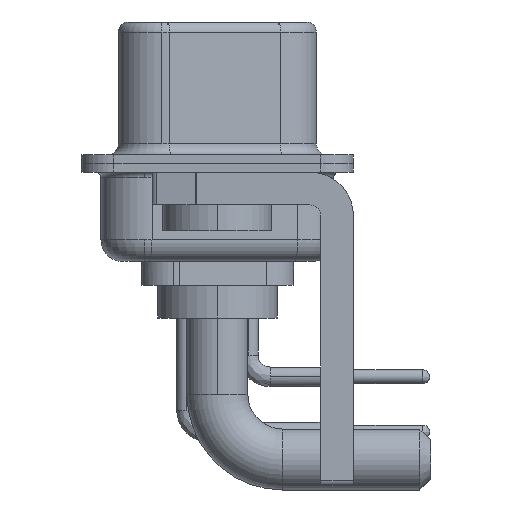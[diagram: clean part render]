
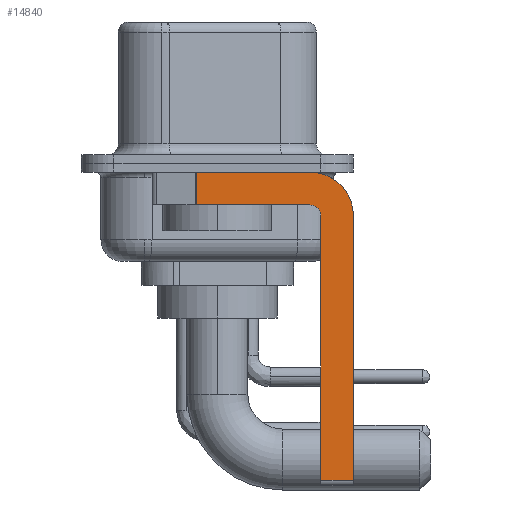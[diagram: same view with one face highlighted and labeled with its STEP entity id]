
A CAD part, left-side view. The second image highlights one B-rep face of the part: STEP entity #14840.
In plain terms, the highlighted planar face has unit normal (-1, 0, 0).
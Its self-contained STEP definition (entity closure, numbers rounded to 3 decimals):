
#221 = DIRECTION ( 'NONE',  ( 1., 0., 0. ) ) ;
#790 = CARTESIAN_POINT ( 'NONE',  ( -2.9, -6.25, -2.4 ) ) ;
#936 = VECTOR ( 'NONE', #21376, 1000. ) ;
#1377 = CARTESIAN_POINT ( 'NONE',  ( -2.9, 0.978, -1.9 ) ) ;
#1381 = EDGE_CURVE ( 'NONE', #5616, #22629, #3759, .T. ) ;
#2346 = CARTESIAN_POINT ( 'NONE',  ( -2.9, -4.25, -14.55 ) ) ;
#3312 = DIRECTION ( 'NONE',  ( -1., 0., 0. ) ) ;
#3759 = LINE ( 'NONE', #8976, #4084 ) ;
#4084 = VECTOR ( 'NONE', #14993, 1000. ) ;
#4318 = DIRECTION ( 'NONE',  ( 1., 0., 0. ) ) ;
#4462 = PLANE ( 'NONE',  #18272 ) ;
#4509 = EDGE_CURVE ( 'NONE', #5616, #27967, #28667, .T. ) ;
#4583 = VERTEX_POINT ( 'NONE', #25008 ) ;
#4845 = ORIENTED_EDGE ( 'NONE', *, *, #4509, .T. ) ;
#5005 = EDGE_CURVE ( 'NONE', #4583, #9487, #27303, .T. ) ;
#5616 = VERTEX_POINT ( 'NONE', #20898 ) ;
#5806 = DIRECTION ( 'NONE',  ( 0., 0., 1. ) ) ;
#6134 = VERTEX_POINT ( 'NONE', #6640 ) ;
#6640 = CARTESIAN_POINT ( 'NONE',  ( -2.9, -4.25, -1.9 ) ) ;
#6803 = ORIENTED_EDGE ( 'NONE', *, *, #7762, .F. ) ;
#7762 = EDGE_CURVE ( 'NONE', #22629, #6134, #23045, .T. ) ;
#8836 = EDGE_CURVE ( 'NONE', #6134, #22430, #11476, .T. ) ;
#8976 = CARTESIAN_POINT ( 'NONE',  ( -2.9, -4.75, -14.8 ) ) ;
#8994 = CARTESIAN_POINT ( 'NONE',  ( -2.9, -4.25, -1.9 ) ) ;
#9487 = VERTEX_POINT ( 'NONE', #790 ) ;
#9536 = AXIS2_PLACEMENT_3D ( 'NONE', #18015, #221, #27249 ) ;
#9842 = CARTESIAN_POINT ( 'NONE',  ( -2.9, -6.25, -2.4 ) ) ;
#10227 = ORIENTED_EDGE ( 'NONE', *, *, #24473, .T. ) ;
#10482 = VECTOR ( 'NONE', #20226, 1000. ) ;
#10531 = EDGE_CURVE ( 'NONE', #9487, #27967, #16999, .T. ) ;
#10676 = ORIENTED_EDGE ( 'NONE', *, *, #1381, .F. ) ;
#11387 = CARTESIAN_POINT ( 'NONE',  ( -2.9, -4.75, -2.4 ) ) ;
#11476 = LINE ( 'NONE', #8994, #10482 ) ;
#13477 = ORIENTED_EDGE ( 'NONE', *, *, #10531, .F. ) ;
#13500 = DIRECTION ( 'NONE',  ( 0., 0., -1. ) ) ;
#13655 = CARTESIAN_POINT ( 'NONE',  ( -2.9, -4.25, -2.4 ) ) ;
#14076 = CARTESIAN_POINT ( 'NONE',  ( -2.9, 3., -0.4 ) ) ;
#14182 = AXIS2_PLACEMENT_3D ( 'NONE', #25821, #3312, #5806 ) ;
#14460 = CARTESIAN_POINT ( 'NONE',  ( -2.9, 0.978, -1.9 ) ) ;
#14488 = LINE ( 'NONE', #14076, #15548 ) ;
#14495 = LINE ( 'NONE', #1377, #936 ) ;
#14840 = ADVANCED_FACE ( 'NONE', ( #26394 ), #4462, .F. ) ;
#14993 = DIRECTION ( 'NONE',  ( 0., 0., 1. ) ) ;
#15467 = CARTESIAN_POINT ( 'NONE',  ( -2.9, 0.978, -0.4 ) ) ;
#15548 = VECTOR ( 'NONE', #23266, 1000. ) ;
#16999 = LINE ( 'NONE', #9842, #26634 ) ;
#17300 = ORIENTED_EDGE ( 'NONE', *, *, #8836, .F. ) ;
#17381 = ORIENTED_EDGE ( 'NONE', *, *, #5005, .F. ) ;
#17556 = EDGE_CURVE ( 'NONE', #22738, #4583, #14488, .T. ) ;
#18015 = CARTESIAN_POINT ( 'NONE',  ( -2.9, -4.25, -2.4 ) ) ;
#18272 = AXIS2_PLACEMENT_3D ( 'NONE', #13655, #4318, #13500 ) ;
#19333 = DIRECTION ( 'NONE',  ( 0., 0., -1. ) ) ;
#19399 = VECTOR ( 'NONE', #22068, 1000. ) ;
#20226 = DIRECTION ( 'NONE',  ( 0., 1., 0. ) ) ;
#20560 = EDGE_LOOP ( 'NONE', ( #28863, #10227, #17300, #6803, #10676, #4845, #13477, #17381 ) ) ;
#20898 = CARTESIAN_POINT ( 'NONE',  ( -2.9, -4.75, -14.55 ) ) ;
#21376 = DIRECTION ( 'NONE',  ( 0., 0., -1. ) ) ;
#22068 = DIRECTION ( 'NONE',  ( 0., -1., 0. ) ) ;
#22430 = VERTEX_POINT ( 'NONE', #14460 ) ;
#22629 = VERTEX_POINT ( 'NONE', #11387 ) ;
#22738 = VERTEX_POINT ( 'NONE', #15467 ) ;
#23045 = CIRCLE ( 'NONE', #14182, 0.5 ) ;
#23266 = DIRECTION ( 'NONE',  ( 0., -1., 0. ) ) ;
#24473 = EDGE_CURVE ( 'NONE', #22738, #22430, #14495, .T. ) ;
#25008 = CARTESIAN_POINT ( 'NONE',  ( -2.9, -4.25, -0.4 ) ) ;
#25821 = CARTESIAN_POINT ( 'NONE',  ( -2.9, -4.25, -2.4 ) ) ;
#26394 = FACE_OUTER_BOUND ( 'NONE', #20560, .T. ) ;
#26634 = VECTOR ( 'NONE', #19333, 1000. ) ;
#27249 = DIRECTION ( 'NONE',  ( 0., 0., -1. ) ) ;
#27303 = CIRCLE ( 'NONE', #9536, 2. ) ;
#27967 = VERTEX_POINT ( 'NONE', #28020 ) ;
#28020 = CARTESIAN_POINT ( 'NONE',  ( -2.9, -6.25, -14.55 ) ) ;
#28667 = LINE ( 'NONE', #2346, #19399 ) ;
#28863 = ORIENTED_EDGE ( 'NONE', *, *, #17556, .F. ) ;
